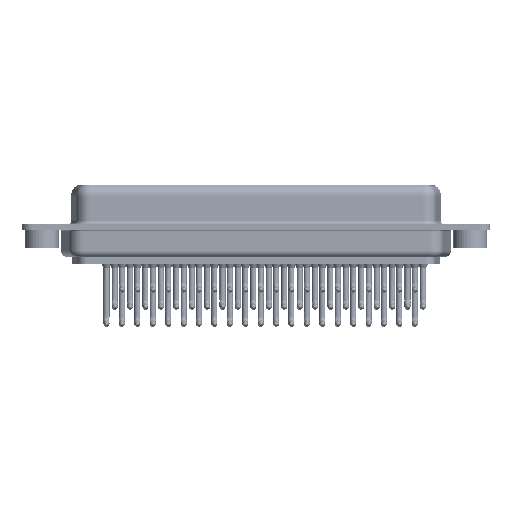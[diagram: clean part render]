
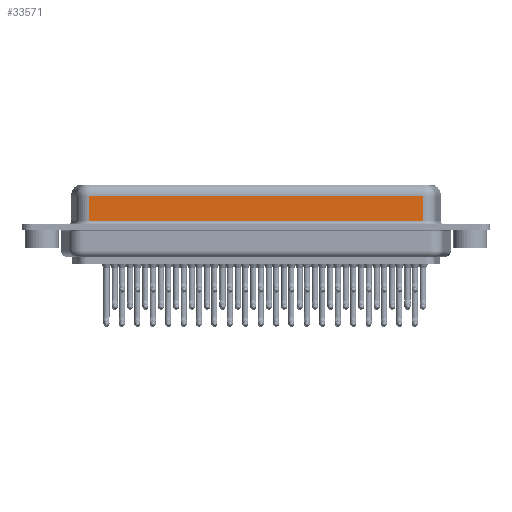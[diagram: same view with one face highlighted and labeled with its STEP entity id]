
A CAD part, front view. The second image highlights one B-rep face of the part: STEP entity #33571.
In plain terms, the highlighted planar face has unit normal (0, -1, 0).
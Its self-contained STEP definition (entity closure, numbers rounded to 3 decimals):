
#6108 = CARTESIAN_POINT ( 'NONE',  ( 56.462, -3.95, 6.4 ) ) ;
#6434 = ORIENTED_EDGE ( 'NONE', *, *, #15574, .T. ) ;
#6946 = LINE ( 'NONE', #13527, #20676 ) ;
#8000 = VERTEX_POINT ( 'NONE', #36470 ) ;
#9575 = CARTESIAN_POINT ( 'NONE',  ( 56.462, -3.95, 0.9 ) ) ;
#9670 = VECTOR ( 'NONE', #26646, 1000. ) ;
#11112 = ORIENTED_EDGE ( 'NONE', *, *, #25798, .T. ) ;
#11692 = PLANE ( 'NONE',  #20449 ) ;
#13527 = CARTESIAN_POINT ( 'NONE',  ( 56.462, -3.95, 4.65 ) ) ;
#14413 = VERTEX_POINT ( 'NONE', #23438 ) ;
#15574 = EDGE_CURVE ( 'NONE', #8000, #17412, #32545, .T. ) ;
#16143 = EDGE_LOOP ( 'NONE', ( #27643, #30800, #6434, #11112 ) ) ;
#16259 = VECTOR ( 'NONE', #21453, 1000. ) ;
#17412 = VERTEX_POINT ( 'NONE', #30485 ) ;
#17545 = DIRECTION ( 'NONE',  ( 0., 0., 1. ) ) ;
#17666 = CARTESIAN_POINT ( 'NONE',  ( 7.038, -3.95, 6.4 ) ) ;
#20449 = AXIS2_PLACEMENT_3D ( 'NONE', #32262, #35247, #17545 ) ;
#20676 = VECTOR ( 'NONE', #36961, 1000. ) ;
#21121 = FACE_OUTER_BOUND ( 'NONE', #16143, .T. ) ;
#21453 = DIRECTION ( 'NONE',  ( 1., 0., 0. ) ) ;
#21620 = VERTEX_POINT ( 'NONE', #24881 ) ;
#21982 = EDGE_CURVE ( 'NONE', #21620, #14413, #26175, .T. ) ;
#23438 = CARTESIAN_POINT ( 'NONE',  ( 56.462, -3.95, 0.9 ) ) ;
#24881 = CARTESIAN_POINT ( 'NONE',  ( 56.462, -3.95, 4.65 ) ) ;
#25053 = LINE ( 'NONE', #9575, #16259 ) ;
#25798 = EDGE_CURVE ( 'NONE', #17412, #14413, #25053, .T. ) ;
#26175 = LINE ( 'NONE', #6108, #9670 ) ;
#26646 = DIRECTION ( 'NONE',  ( 0., 0., -1. ) ) ;
#27643 = ORIENTED_EDGE ( 'NONE', *, *, #21982, .F. ) ;
#28837 = EDGE_CURVE ( 'NONE', #21620, #8000, #6946, .T. ) ;
#29543 = DIRECTION ( 'NONE',  ( 0., 0., -1. ) ) ;
#30485 = CARTESIAN_POINT ( 'NONE',  ( 7.038, -3.95, 0.9 ) ) ;
#30800 = ORIENTED_EDGE ( 'NONE', *, *, #28837, .T. ) ;
#31594 = VECTOR ( 'NONE', #29543, 1000. ) ;
#32262 = CARTESIAN_POINT ( 'NONE',  ( 56.462, -3.95, 6.4 ) ) ;
#32545 = LINE ( 'NONE', #17666, #31594 ) ;
#33571 = ADVANCED_FACE ( 'NONE', ( #21121 ), #11692, .F. ) ;
#35247 = DIRECTION ( 'NONE',  ( 0., 1., 0. ) ) ;
#36470 = CARTESIAN_POINT ( 'NONE',  ( 7.038, -3.95, 4.65 ) ) ;
#36961 = DIRECTION ( 'NONE',  ( -1., 0., 0. ) ) ;
